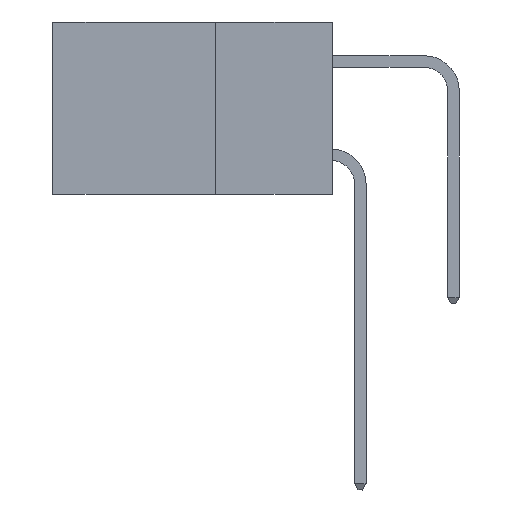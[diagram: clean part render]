
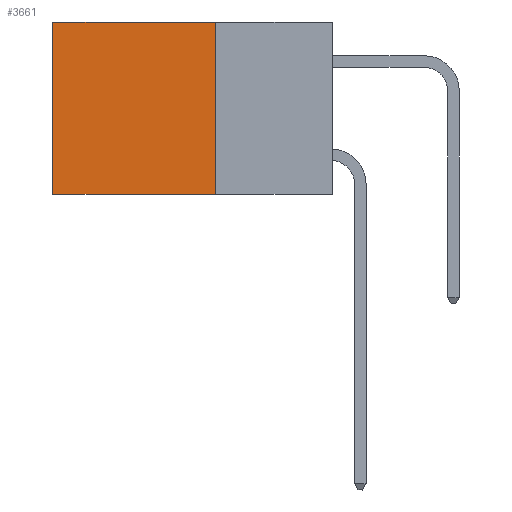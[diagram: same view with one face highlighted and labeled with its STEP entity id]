
A CAD part, left-side view. The second image highlights one B-rep face of the part: STEP entity #3661.
In plain terms, the highlighted planar face has unit normal (-1, 0, 0).
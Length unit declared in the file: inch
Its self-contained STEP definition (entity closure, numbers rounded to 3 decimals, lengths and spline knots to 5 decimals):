
#727 = ORIENTED_EDGE ( 'NONE', *, *, #888, .T. ) ;
#745 = FACE_OUTER_BOUND ( 'NONE', #9743, .T. ) ;
#874 = DIRECTION ( 'NONE',  ( 0., 0., -1. ) ) ;
#888 = EDGE_CURVE ( 'NONE', #6885, #12386, #8378, .T. ) ;
#1047 = VERTEX_POINT ( 'NONE', #7836 ) ;
#1401 = CARTESIAN_POINT ( 'NONE',  ( 0.2615, 0.25, 0. ) ) ;
#2131 = LINE ( 'NONE', #6034, #7092 ) ;
#3251 = DIRECTION ( 'NONE',  ( 0., 1., 0. ) ) ;
#3661 = ADVANCED_FACE ( 'NONE', ( #745 ), #10600, .F. ) ;
#3764 = DIRECTION ( 'NONE',  ( 0., 0., -1. ) ) ;
#4924 = ORIENTED_EDGE ( 'NONE', *, *, #9574, .T. ) ;
#5002 = VECTOR ( 'NONE', #3764, 39.37008 ) ;
#5054 = CARTESIAN_POINT ( 'NONE',  ( 0.2615, 0.25, -0.37 ) ) ;
#5638 = CARTESIAN_POINT ( 'NONE',  ( 0.2615, 0.25, -0.37 ) ) ;
#6034 = CARTESIAN_POINT ( 'NONE',  ( 0.2615, 0.25, 0. ) ) ;
#6472 = VECTOR ( 'NONE', #8505, 39.37008 ) ;
#6885 = VERTEX_POINT ( 'NONE', #10009 ) ;
#7092 = VECTOR ( 'NONE', #3251, 39.37008 ) ;
#7836 = CARTESIAN_POINT ( 'NONE',  ( 0.2615, 0.25, -0.37 ) ) ;
#8378 = LINE ( 'NONE', #10273, #6472 ) ;
#8496 = CARTESIAN_POINT ( 'NONE',  ( 0.2615, 0.25, -0.37 ) ) ;
#8505 = DIRECTION ( 'NONE',  ( 0., 0., -1. ) ) ;
#8522 = EDGE_CURVE ( 'NONE', #9267, #1047, #9615, .T. ) ;
#8791 = ORIENTED_EDGE ( 'NONE', *, *, #12096, .F. ) ;
#9267 = VERTEX_POINT ( 'NONE', #1401 ) ;
#9574 = EDGE_CURVE ( 'NONE', #9267, #6885, #2131, .T. ) ;
#9615 = LINE ( 'NONE', #8496, #5002 ) ;
#9694 = CARTESIAN_POINT ( 'NONE',  ( 0.2615, 0.6, -0.37 ) ) ;
#9743 = EDGE_LOOP ( 'NONE', ( #727, #8791, #11193, #4924 ) ) ;
#10009 = CARTESIAN_POINT ( 'NONE',  ( 0.2615, 0.6, 0. ) ) ;
#10080 = DIRECTION ( 'NONE',  ( 0., 1., 0. ) ) ;
#10273 = CARTESIAN_POINT ( 'NONE',  ( 0.2615, 0.6, -0.37 ) ) ;
#10572 = AXIS2_PLACEMENT_3D ( 'NONE', #5638, #12692, #874 ) ;
#10600 = PLANE ( 'NONE',  #10572 ) ;
#10887 = VECTOR ( 'NONE', #10080, 39.37008 ) ;
#11193 = ORIENTED_EDGE ( 'NONE', *, *, #8522, .F. ) ;
#11908 = LINE ( 'NONE', #5054, #10887 ) ;
#12096 = EDGE_CURVE ( 'NONE', #1047, #12386, #11908, .T. ) ;
#12386 = VERTEX_POINT ( 'NONE', #9694 ) ;
#12692 = DIRECTION ( 'NONE',  ( 1., 0., 0. ) ) ;
